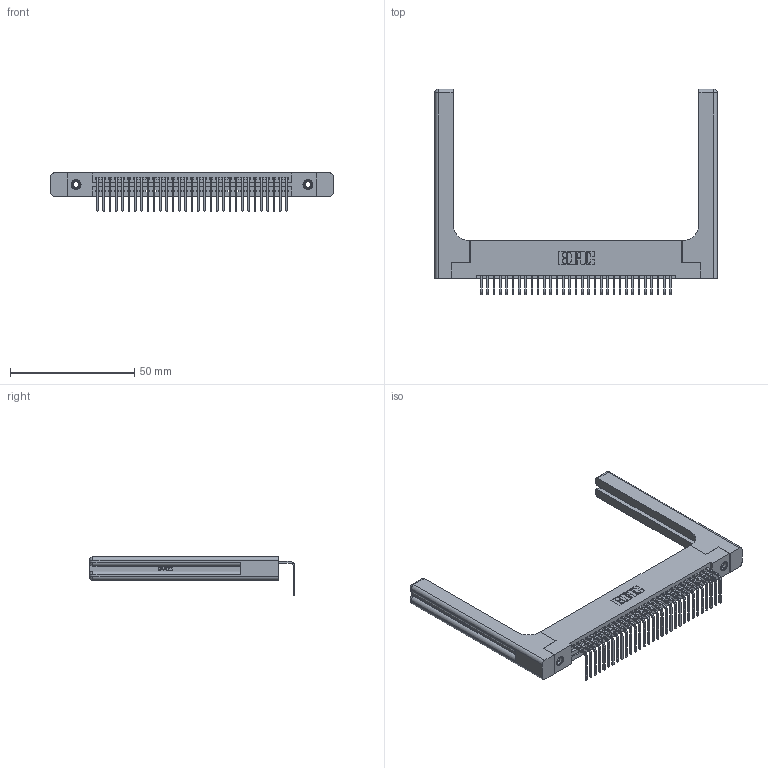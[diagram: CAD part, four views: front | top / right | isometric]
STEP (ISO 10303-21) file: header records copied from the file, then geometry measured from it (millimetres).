
FILE_DESCRIPTION (( 'STEP AP203' ), '1' );
FILE_NAME ('345-031-558-158.STEP', '2019-10-10T14:23:31', ( '' ), ( '' ), 'SwSTEP 2.0', 'SolidWorks 2016', '' );
FILE_SCHEMA (( 'CONFIG_CONTROL_DESIGN' ));
Length unit declared in the file: inch
Products named in the file (5): 345-250-001_345-250-001-102; 345-220-058_345-220-058; 345-031-558-158; 345 Part_Flush Mounting Lugs - 0.156 Dia-TH; 345-292-001_558 Tail - 2
Assembly tree (36 placements, depth 2):
  345-031-558-158
    345 Part_Flush Mounting Lugs - 0.156 Dia-TH
    345-292-001_558 Tail - 2  x31
    345-250-001_345-250-001-102  x2
    345-220-058_345-220-058  x2
Bounding box: 113.77 x 82.79 x 15.37 mm (x, y, z)
Volume: 19323.8 mm3; surface area: 20140.2 mm2
Topology: 36 solids, 36 shells, 2242 faces, 6649 edges, 4370 vertices
Faces by surface type: plane 1530, cylinder 652, bspline 36, cone 12, sphere 8, torus 4
Entity records: 30078 total; most frequent: CARTESIAN_POINT 6182, ORIENTED_EDGE 4944, DIRECTION 4362, EDGE_CURVE 2472, LINE 2124, VECTOR 2124, VERTEX_POINT 1638, AXIS2_PLACEMENT_3D 1119
